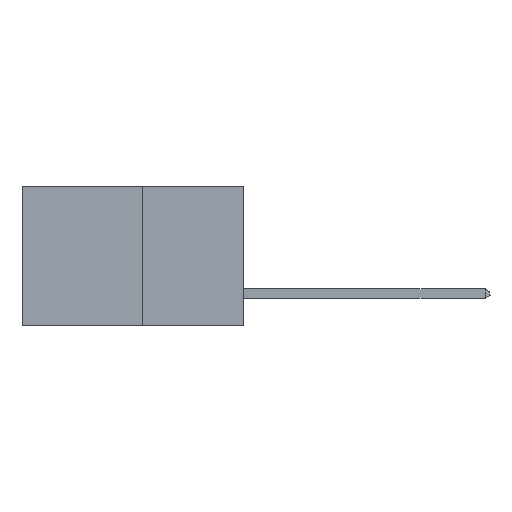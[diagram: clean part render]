
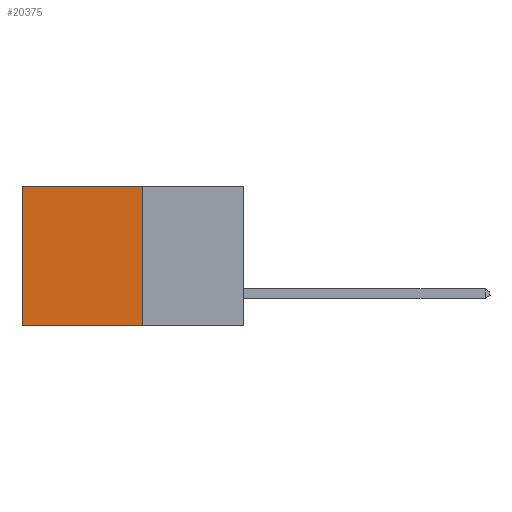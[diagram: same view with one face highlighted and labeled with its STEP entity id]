
A CAD part, left-side view. The second image highlights one B-rep face of the part: STEP entity #20375.
In plain terms, the highlighted planar face has unit normal (-1, 0, 0).
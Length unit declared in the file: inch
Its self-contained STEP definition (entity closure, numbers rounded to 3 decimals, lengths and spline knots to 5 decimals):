
#1 = LINE ( 'NONE', #17322, #16432 ) ;
#237 = LINE ( 'NONE', #18521, #2343 ) ;
#1346 = ORIENTED_EDGE ( 'NONE', *, *, #16190, .F. ) ;
#1842 = EDGE_CURVE ( 'NONE', #17539, #9328, #237, .T. ) ;
#2026 = CARTESIAN_POINT ( 'NONE',  ( 0.277, 0.59, -0.37 ) ) ;
#2258 = AXIS2_PLACEMENT_3D ( 'NONE', #18337, #19873, #10655 ) ;
#2343 = VECTOR ( 'NONE', #17854, 39.37008 ) ;
#2774 = CARTESIAN_POINT ( 'NONE',  ( 0.277, 0.27, -0.37 ) ) ;
#3286 = VERTEX_POINT ( 'NONE', #2026 ) ;
#3318 = EDGE_CURVE ( 'NONE', #17539, #7785, #19721, .T. ) ;
#3526 = CARTESIAN_POINT ( 'NONE',  ( 0.277, 0.27, 0. ) ) ;
#3652 = LINE ( 'NONE', #14100, #19288 ) ;
#5337 = EDGE_LOOP ( 'NONE', ( #6839, #1346, #15064, #17589 ) ) ;
#6839 = ORIENTED_EDGE ( 'NONE', *, *, #19916, .T. ) ;
#6908 = FACE_OUTER_BOUND ( 'NONE', #5337, .T. ) ;
#7785 = VERTEX_POINT ( 'NONE', #15485 ) ;
#9328 = VERTEX_POINT ( 'NONE', #19053 ) ;
#10655 = DIRECTION ( 'NONE',  ( 0., 0., -1. ) ) ;
#11045 = VECTOR ( 'NONE', #19940, 39.37008 ) ;
#12715 = DIRECTION ( 'NONE',  ( 0., 1., 0. ) ) ;
#14100 = CARTESIAN_POINT ( 'NONE',  ( 0.277, 0.59, -0.37 ) ) ;
#15064 = ORIENTED_EDGE ( 'NONE', *, *, #3318, .F. ) ;
#15485 = CARTESIAN_POINT ( 'NONE',  ( 0.277, 0.27, -0.37 ) ) ;
#16190 = EDGE_CURVE ( 'NONE', #7785, #3286, #1, .T. ) ;
#16432 = VECTOR ( 'NONE', #12715, 39.37008 ) ;
#16823 = PLANE ( 'NONE',  #2258 ) ;
#17163 = DIRECTION ( 'NONE',  ( 0., 0., -1. ) ) ;
#17322 = CARTESIAN_POINT ( 'NONE',  ( 0.277, 0.27, -0.37 ) ) ;
#17539 = VERTEX_POINT ( 'NONE', #3526 ) ;
#17589 = ORIENTED_EDGE ( 'NONE', *, *, #1842, .T. ) ;
#17854 = DIRECTION ( 'NONE',  ( 0., 1., 0. ) ) ;
#18337 = CARTESIAN_POINT ( 'NONE',  ( 0.277, 0.27, -0.37 ) ) ;
#18521 = CARTESIAN_POINT ( 'NONE',  ( 0.277, 0.27, 0. ) ) ;
#19053 = CARTESIAN_POINT ( 'NONE',  ( 0.277, 0.59, 0. ) ) ;
#19288 = VECTOR ( 'NONE', #17163, 39.37008 ) ;
#19721 = LINE ( 'NONE', #2774, #11045 ) ;
#19873 = DIRECTION ( 'NONE',  ( 1., 0., 0. ) ) ;
#19916 = EDGE_CURVE ( 'NONE', #9328, #3286, #3652, .T. ) ;
#19940 = DIRECTION ( 'NONE',  ( 0., 0., -1. ) ) ;
#20375 = ADVANCED_FACE ( 'NONE', ( #6908 ), #16823, .F. ) ;
